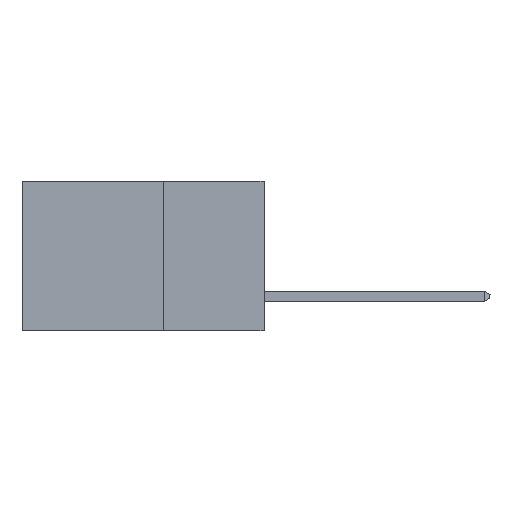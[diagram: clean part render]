
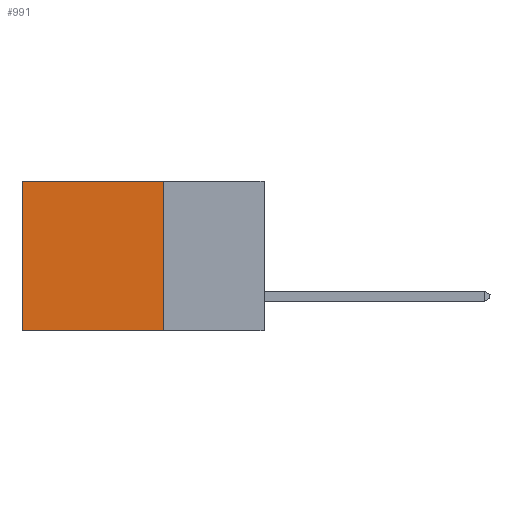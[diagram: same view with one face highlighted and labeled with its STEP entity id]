
A CAD part, left-side view. The second image highlights one B-rep face of the part: STEP entity #991.
In plain terms, the highlighted planar face has unit normal (-1, 0, 0).
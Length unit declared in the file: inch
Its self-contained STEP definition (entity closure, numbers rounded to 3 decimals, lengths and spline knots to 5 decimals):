
#548 = LINE ( 'NONE', #5855, #3728 ) ;
#991 = ADVANCED_FACE ( 'NONE', ( #1772 ), #22765, .F. ) ;
#1772 = FACE_OUTER_BOUND ( 'NONE', #17971, .T. ) ;
#2630 = DIRECTION ( 'NONE',  ( 0., 0., -1. ) ) ;
#3654 = EDGE_CURVE ( 'NONE', #12945, #3764, #548, .T. ) ;
#3728 = VECTOR ( 'NONE', #7897, 39.37008 ) ;
#3764 = VERTEX_POINT ( 'NONE', #10315 ) ;
#3944 = VECTOR ( 'NONE', #10349, 39.37008 ) ;
#4273 = DIRECTION ( 'NONE',  ( 0., 0., -1. ) ) ;
#4575 = CARTESIAN_POINT ( 'NONE',  ( 0.2615, 0.25, -0.37 ) ) ;
#4690 = LINE ( 'NONE', #4575, #3944 ) ;
#5855 = CARTESIAN_POINT ( 'NONE',  ( 0.2615, 0.25, 0. ) ) ;
#6465 = LINE ( 'NONE', #22948, #12880 ) ;
#7897 = DIRECTION ( 'NONE',  ( 0., 1., 0. ) ) ;
#9114 = DIRECTION ( 'NONE',  ( 1., 0., 0. ) ) ;
#10023 = EDGE_CURVE ( 'NONE', #10976, #11639, #4690, .T. ) ;
#10315 = CARTESIAN_POINT ( 'NONE',  ( 0.2615, 0.6, 0. ) ) ;
#10349 = DIRECTION ( 'NONE',  ( 0., 1., 0. ) ) ;
#10976 = VERTEX_POINT ( 'NONE', #13874 ) ;
#11536 = CARTESIAN_POINT ( 'NONE',  ( 0.2615, 0.25, 0. ) ) ;
#11639 = VERTEX_POINT ( 'NONE', #14898 ) ;
#12880 = VECTOR ( 'NONE', #17285, 39.37008 ) ;
#12945 = VERTEX_POINT ( 'NONE', #11536 ) ;
#13469 = LINE ( 'NONE', #22708, #21781 ) ;
#13874 = CARTESIAN_POINT ( 'NONE',  ( 0.2615, 0.25, -0.37 ) ) ;
#14111 = ORIENTED_EDGE ( 'NONE', *, *, #17635, .F. ) ;
#14121 = EDGE_CURVE ( 'NONE', #3764, #11639, #6465, .T. ) ;
#14279 = ORIENTED_EDGE ( 'NONE', *, *, #3654, .T. ) ;
#14898 = CARTESIAN_POINT ( 'NONE',  ( 0.2615, 0.6, -0.37 ) ) ;
#17285 = DIRECTION ( 'NONE',  ( 0., 0., -1. ) ) ;
#17635 = EDGE_CURVE ( 'NONE', #12945, #10976, #13469, .T. ) ;
#17971 = EDGE_LOOP ( 'NONE', ( #22634, #19135, #14111, #14279 ) ) ;
#19135 = ORIENTED_EDGE ( 'NONE', *, *, #10023, .F. ) ;
#20137 = CARTESIAN_POINT ( 'NONE',  ( 0.2615, 0.25, -0.37 ) ) ;
#20391 = AXIS2_PLACEMENT_3D ( 'NONE', #20137, #9114, #4273 ) ;
#21781 = VECTOR ( 'NONE', #2630, 39.37008 ) ;
#22634 = ORIENTED_EDGE ( 'NONE', *, *, #14121, .T. ) ;
#22708 = CARTESIAN_POINT ( 'NONE',  ( 0.2615, 0.25, -0.37 ) ) ;
#22765 = PLANE ( 'NONE',  #20391 ) ;
#22948 = CARTESIAN_POINT ( 'NONE',  ( 0.2615, 0.6, -0.37 ) ) ;
